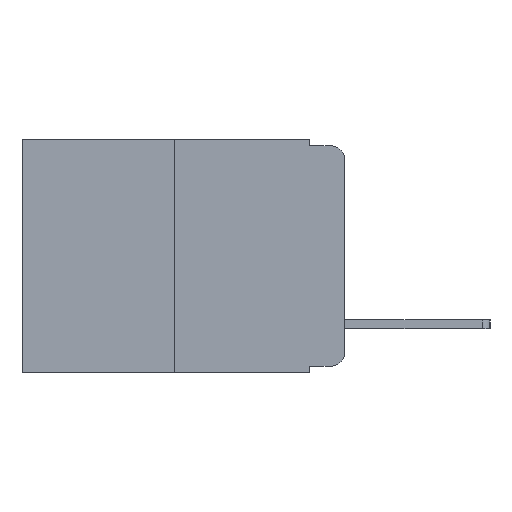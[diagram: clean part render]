
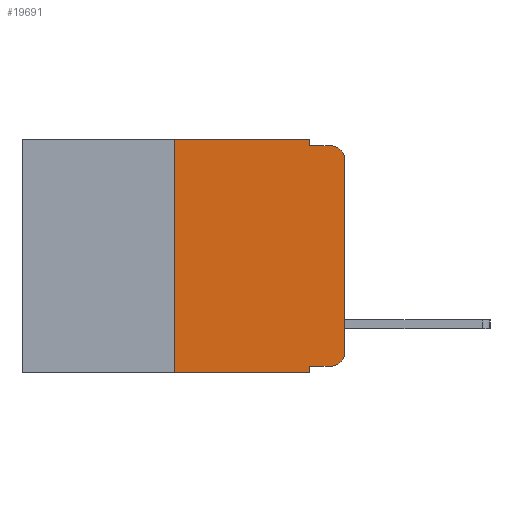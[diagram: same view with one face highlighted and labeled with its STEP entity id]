
A CAD part, left-side view. The second image highlights one B-rep face of the part: STEP entity #19691.
In plain terms, the highlighted planar face has unit normal (-1, 0, 0).
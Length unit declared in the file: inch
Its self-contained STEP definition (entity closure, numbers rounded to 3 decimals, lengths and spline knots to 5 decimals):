
#67 = ORIENTED_EDGE ( 'NONE', *, *, #17786, .F. ) ;
#256 = ORIENTED_EDGE ( 'NONE', *, *, #2286, .T. ) ;
#359 = EDGE_CURVE ( 'NONE', #19457, #21084, #13294, .T. ) ;
#593 = DIRECTION ( 'NONE',  ( 0., -1., 0. ) ) ;
#725 = LINE ( 'NONE', #5547, #14338 ) ;
#1206 = DIRECTION ( 'NONE',  ( 0., 0., -1. ) ) ;
#1522 = VERTEX_POINT ( 'NONE', #7356 ) ;
#2018 = DIRECTION ( 'NONE',  ( 0., -1., 0. ) ) ;
#2193 = ORIENTED_EDGE ( 'NONE', *, *, #359, .F. ) ;
#2195 = LINE ( 'NONE', #8949, #15155 ) ;
#2242 = VECTOR ( 'NONE', #10491, 39.37008 ) ;
#2286 = EDGE_CURVE ( 'NONE', #14476, #8790, #4482, .T. ) ;
#2412 = VECTOR ( 'NONE', #21514, 39.37008 ) ;
#2431 = VERTEX_POINT ( 'NONE', #11615 ) ;
#2670 = DIRECTION ( 'NONE',  ( -1., 0., 0. ) ) ;
#2724 = CARTESIAN_POINT ( 'NONE',  ( 0., 0.051, 0. ) ) ;
#2834 = EDGE_LOOP ( 'NONE', ( #17716, #256, #17197, #21557, #67, #10486, #18208, #2193, #5716, #9180 ) ) ;
#3775 = VECTOR ( 'NONE', #1206, 39.37008 ) ;
#4475 = DIRECTION ( 'NONE',  ( 0., 0., -1. ) ) ;
#4482 = CIRCLE ( 'NONE', #16718, 0.02 ) ;
#4563 = LINE ( 'NONE', #2724, #13017 ) ;
#4657 = CARTESIAN_POINT ( 'NONE',  ( 0., 0., -0.03 ) ) ;
#5547 = CARTESIAN_POINT ( 'NONE',  ( 0., 0., 0. ) ) ;
#5716 = ORIENTED_EDGE ( 'NONE', *, *, #12714, .T. ) ;
#5782 = DIRECTION ( 'NONE',  ( 0., 0., -1. ) ) ;
#5806 = CARTESIAN_POINT ( 'NONE',  ( 0., 0.473, -0.343 ) ) ;
#5933 = VERTEX_POINT ( 'NONE', #9763 ) ;
#6391 = CARTESIAN_POINT ( 'NONE',  ( 0., 0.02, -0.03 ) ) ;
#6471 = LINE ( 'NONE', #19872, #2412 ) ;
#7106 = CARTESIAN_POINT ( 'NONE',  ( 0., 0.25, 0. ) ) ;
#7354 = CARTESIAN_POINT ( 'NONE',  ( 0., 0.051, -0.01 ) ) ;
#7356 = CARTESIAN_POINT ( 'NONE',  ( 0., 0.02, -0.333 ) ) ;
#7952 = CARTESIAN_POINT ( 'NONE',  ( 0., 0.051, 0. ) ) ;
#8040 = FACE_OUTER_BOUND ( 'NONE', #2834, .T. ) ;
#8312 = CARTESIAN_POINT ( 'NONE',  ( 0., 0.051, -0.333 ) ) ;
#8691 = AXIS2_PLACEMENT_3D ( 'NONE', #12855, #2670, #14517 ) ;
#8790 = VERTEX_POINT ( 'NONE', #20305 ) ;
#8949 = CARTESIAN_POINT ( 'NONE',  ( 0., 0.473, 0. ) ) ;
#8953 = EDGE_CURVE ( 'NONE', #1522, #20530, #21518, .T. ) ;
#9180 = ORIENTED_EDGE ( 'NONE', *, *, #8953, .T. ) ;
#9763 = CARTESIAN_POINT ( 'NONE',  ( 0., 0.25, 0. ) ) ;
#9770 = CARTESIAN_POINT ( 'NONE',  ( 0., 0.051, 0. ) ) ;
#9836 = DIRECTION ( 'NONE',  ( 1., 0., 0. ) ) ;
#10010 = DIRECTION ( 'NONE',  ( 0., -1., 0. ) ) ;
#10459 = CARTESIAN_POINT ( 'NONE',  ( 0., 0., -0.313 ) ) ;
#10486 = ORIENTED_EDGE ( 'NONE', *, *, #12289, .F. ) ;
#10491 = DIRECTION ( 'NONE',  ( 0., 0., 1. ) ) ;
#11184 = EDGE_CURVE ( 'NONE', #2431, #21084, #18588, .T. ) ;
#11615 = CARTESIAN_POINT ( 'NONE',  ( 0., 0.25, -0.343 ) ) ;
#12095 = PLANE ( 'NONE',  #12317 ) ;
#12289 = EDGE_CURVE ( 'NONE', #2431, #5933, #20059, .T. ) ;
#12317 = AXIS2_PLACEMENT_3D ( 'NONE', #19701, #9836, #21344 ) ;
#12714 = EDGE_CURVE ( 'NONE', #19457, #1522, #20037, .T. ) ;
#12855 = CARTESIAN_POINT ( 'NONE',  ( 0., 0.02, -0.313 ) ) ;
#13017 = VECTOR ( 'NONE', #4475, 39.37008 ) ;
#13218 = VERTEX_POINT ( 'NONE', #9770 ) ;
#13294 = LINE ( 'NONE', #7952, #3775 ) ;
#14338 = VECTOR ( 'NONE', #17192, 39.37008 ) ;
#14476 = VERTEX_POINT ( 'NONE', #4657 ) ;
#14517 = DIRECTION ( 'NONE',  ( 0., 0., -1. ) ) ;
#14760 = EDGE_CURVE ( 'NONE', #20530, #14476, #725, .T. ) ;
#15012 = EDGE_CURVE ( 'NONE', #13218, #21206, #4563, .T. ) ;
#15155 = VECTOR ( 'NONE', #2018, 39.37008 ) ;
#15685 = VECTOR ( 'NONE', #10010, 39.37008 ) ;
#16484 = CARTESIAN_POINT ( 'NONE',  ( 0., 0.051, -0.333 ) ) ;
#16718 = AXIS2_PLACEMENT_3D ( 'NONE', #6391, #18443, #5782 ) ;
#17192 = DIRECTION ( 'NONE',  ( 0., 0., 1. ) ) ;
#17197 = ORIENTED_EDGE ( 'NONE', *, *, #18878, .F. ) ;
#17716 = ORIENTED_EDGE ( 'NONE', *, *, #14760, .T. ) ;
#17786 = EDGE_CURVE ( 'NONE', #5933, #13218, #2195, .T. ) ;
#18071 = VECTOR ( 'NONE', #593, 39.37008 ) ;
#18208 = ORIENTED_EDGE ( 'NONE', *, *, #11184, .T. ) ;
#18443 = DIRECTION ( 'NONE',  ( -1., 0., 0. ) ) ;
#18574 = CARTESIAN_POINT ( 'NONE',  ( 0., 0.051, -0.343 ) ) ;
#18588 = LINE ( 'NONE', #5806, #18071 ) ;
#18878 = EDGE_CURVE ( 'NONE', #21206, #8790, #6471, .T. ) ;
#19457 = VERTEX_POINT ( 'NONE', #16484 ) ;
#19691 = ADVANCED_FACE ( 'NONE', ( #8040 ), #12095, .F. ) ;
#19701 = CARTESIAN_POINT ( 'NONE',  ( 0., 0.473, 0. ) ) ;
#19872 = CARTESIAN_POINT ( 'NONE',  ( 0., 0.051, -0.01 ) ) ;
#20037 = LINE ( 'NONE', #8312, #15685 ) ;
#20059 = LINE ( 'NONE', #7106, #2242 ) ;
#20305 = CARTESIAN_POINT ( 'NONE',  ( 0., 0.02, -0.01 ) ) ;
#20530 = VERTEX_POINT ( 'NONE', #10459 ) ;
#21084 = VERTEX_POINT ( 'NONE', #18574 ) ;
#21206 = VERTEX_POINT ( 'NONE', #7354 ) ;
#21344 = DIRECTION ( 'NONE',  ( 0., 0., -1. ) ) ;
#21514 = DIRECTION ( 'NONE',  ( 0., -1., 0. ) ) ;
#21518 = CIRCLE ( 'NONE', #8691, 0.02 ) ;
#21557 = ORIENTED_EDGE ( 'NONE', *, *, #15012, .F. ) ;
